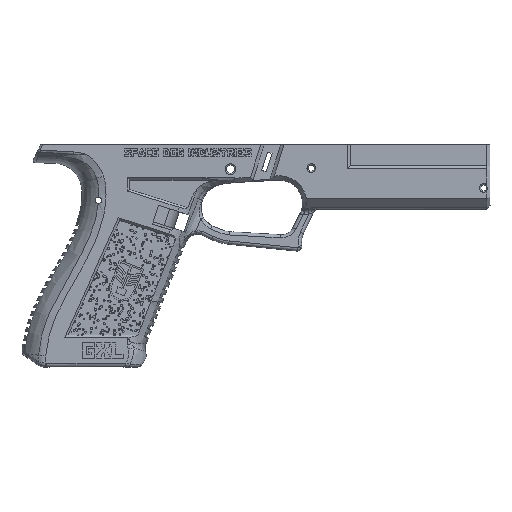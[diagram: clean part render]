
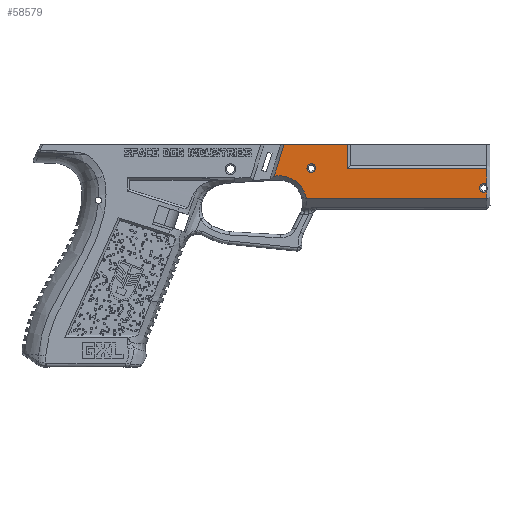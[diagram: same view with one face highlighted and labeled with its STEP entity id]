
A CAD part, top view. The second image highlights one B-rep face of the part: STEP entity #58579.
In plain terms, the highlighted planar face has unit normal (0, 0, 1).
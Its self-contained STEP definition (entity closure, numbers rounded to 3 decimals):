
#2546=FACE_BOUND('',#10763,.T.);
#2971=CIRCLE('',#62154,2.);
#2972=CIRCLE('',#62156,13.);
#2973=CIRCLE('',#62157,2.025);
#7183=FACE_OUTER_BOUND('',#10762,.T.);
#10762=EDGE_LOOP('',(#39445,#39446,#39447,#39448,#39449,#39450,#39451,#39452,
#39453,#39454));
#10763=EDGE_LOOP('',(#39455));
#16110=LINE('',#73279,#19924);
#16142=LINE('',#73619,#19956);
#16143=LINE('',#73621,#19957);
#16144=LINE('',#73622,#19958);
#16145=LINE('',#73624,#19959);
#16146=LINE('',#73626,#19960);
#16147=LINE('',#73630,#19961);
#16148=LINE('',#73631,#19962);
#19924=VECTOR('',#63740,10.);
#19956=VECTOR('',#63786,10.);
#19957=VECTOR('',#63787,10.);
#19958=VECTOR('',#63788,10.);
#19959=VECTOR('',#63789,10.);
#19960=VECTOR('',#63790,10.);
#19961=VECTOR('',#63793,10.);
#19962=VECTOR('',#63794,10.);
#23948=VERTEX_POINT('',#73276);
#23949=VERTEX_POINT('',#73278);
#23982=VERTEX_POINT('',#73591);
#23985=VERTEX_POINT('',#73604);
#23986=VERTEX_POINT('',#73618);
#23987=VERTEX_POINT('',#73620);
#23988=VERTEX_POINT('',#73623);
#23989=VERTEX_POINT('',#73625);
#23990=VERTEX_POINT('',#73627);
#23991=VERTEX_POINT('',#73629);
#23992=VERTEX_POINT('',#73632);
#30091=EDGE_CURVE('',#23948,#23949,#16110,.T.);
#30131=EDGE_CURVE('',#23985,#23982,#2971,.T.);
#30132=EDGE_CURVE('',#23986,#23985,#16142,.T.);
#30133=EDGE_CURVE('',#23986,#23987,#16143,.T.);
#30134=EDGE_CURVE('',#23949,#23987,#16144,.T.);
#30135=EDGE_CURVE('',#23988,#23948,#16145,.T.);
#30136=EDGE_CURVE('',#23989,#23988,#16146,.T.);
#30137=EDGE_CURVE('',#23990,#23989,#2972,.T.);
#30138=EDGE_CURVE('',#23991,#23990,#16147,.T.);
#30139=EDGE_CURVE('',#23982,#23991,#16148,.T.);
#30140=EDGE_CURVE('',#23992,#23992,#2973,.T.);
#39445=ORIENTED_EDGE('',*,*,#30131,.F.);
#39446=ORIENTED_EDGE('',*,*,#30132,.F.);
#39447=ORIENTED_EDGE('',*,*,#30133,.T.);
#39448=ORIENTED_EDGE('',*,*,#30134,.F.);
#39449=ORIENTED_EDGE('',*,*,#30091,.F.);
#39450=ORIENTED_EDGE('',*,*,#30135,.F.);
#39451=ORIENTED_EDGE('',*,*,#30136,.F.);
#39452=ORIENTED_EDGE('',*,*,#30137,.F.);
#39453=ORIENTED_EDGE('',*,*,#30138,.F.);
#39454=ORIENTED_EDGE('',*,*,#30139,.F.);
#39455=ORIENTED_EDGE('',*,*,#30140,.T.);
#57484=PLANE('',#62155);
#58579=ADVANCED_FACE('',(#7183,#2546),#57484,.F.);
#62154=AXIS2_PLACEMENT_3D('',#73616,#63782,#63783);
#62155=AXIS2_PLACEMENT_3D('',#73617,#63784,#63785);
#62156=AXIS2_PLACEMENT_3D('',#73628,#63791,#63792);
#62157=AXIS2_PLACEMENT_3D('',#73633,#63795,#63796);
#63740=DIRECTION('',(1.,0.,0.));
#63782=DIRECTION('center_axis',(0.,0.,
1.));
#63783=DIRECTION('ref_axis',(-1.,0.,0.));
#63784=DIRECTION('center_axis',(0.,0.,
-1.));
#63785=DIRECTION('ref_axis',(0.,1.,0.));
#63786=DIRECTION('',(0.,-1.,0.));
#63787=DIRECTION('',(-1.,0.,0.));
#63788=DIRECTION('',(0.,-1.,0.));
#63789=DIRECTION('',(0.301,0.954,0.));
#63790=DIRECTION('',(-0.999,-0.055,0.));
#63791=DIRECTION('center_axis',(0.,0.,
1.));
#63792=DIRECTION('ref_axis',(0.892,-0.452,0.));
#63793=DIRECTION('',(-1.,0.,0.));
#63794=DIRECTION('',(0.,-1.,0.));
#63795=DIRECTION('center_axis',(0.,0.,
-1.));
#63796=DIRECTION('ref_axis',(0.776,-0.63,0.));
#73276=CARTESIAN_POINT('',(82.591,1.767,-56.855));
#73278=CARTESIAN_POINT('',(112.635,1.767,-56.855));
#73279=CARTESIAN_POINT('',(33.317,1.767,-56.855));
#73591=CARTESIAN_POINT('',(178.635,-20.11,-56.855));
#73604=CARTESIAN_POINT('',(178.635,-17.464,-56.855));
#73616=CARTESIAN_POINT('Origin',(177.135,-18.787,-56.855));
#73617=CARTESIAN_POINT('Origin',(103.31,1.259,-56.855));
#73618=CARTESIAN_POINT('',(178.635,-9.733,-56.855));
#73619=CARTESIAN_POINT('',(178.635,-25.087,-56.855));
#73620=CARTESIAN_POINT('',(112.635,-9.733,-56.855));
#73621=CARTESIAN_POINT('',(105.549,-9.733,-56.855));
#73622=CARTESIAN_POINT('',(112.635,1.513,-56.855));
#73623=CARTESIAN_POINT('',(77.883,-13.165,-56.855));
#73624=CARTESIAN_POINT('',(82.185,0.48,-56.855));
#73625=CARTESIAN_POINT('',(80.217,-13.037,-56.855));
#73626=CARTESIAN_POINT('',(81.633,-12.959,-56.855));
#73627=CARTESIAN_POINT('',(93.078,-23.787,-56.855));
#73628=CARTESIAN_POINT('Origin',(80.274,-26.037,-56.855));
#73629=CARTESIAN_POINT('',(178.635,-23.787,-56.855));
#73630=CARTESIAN_POINT('',(89.618,-23.787,-56.855));
#73631=CARTESIAN_POINT('',(178.635,-25.087,-56.855));
#73632=CARTESIAN_POINT('',(97.469,-9.398,-56.855));
#73633=CARTESIAN_POINT('Origin',(95.444,-9.398,-56.855));
